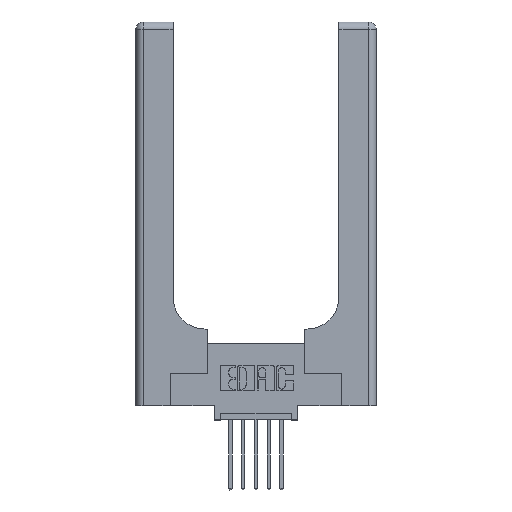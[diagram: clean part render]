
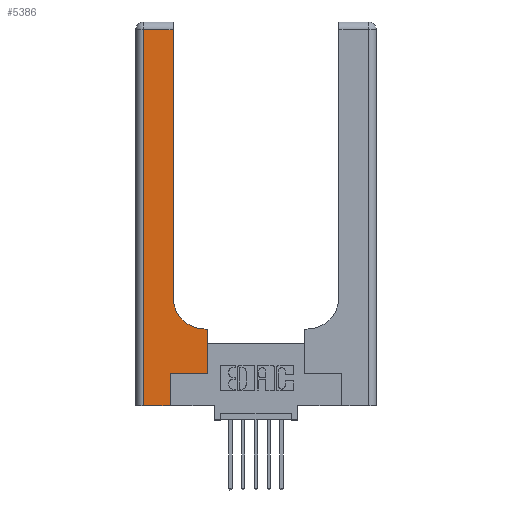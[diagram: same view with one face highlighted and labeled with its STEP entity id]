
A CAD part, top view. The second image highlights one B-rep face of the part: STEP entity #5386.
In plain terms, the highlighted planar face has unit normal (0, 0, 1).
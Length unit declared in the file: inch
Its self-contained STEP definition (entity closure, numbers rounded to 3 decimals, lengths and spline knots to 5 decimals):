
#36 = DIRECTION ( 'NONE',  ( 0., 1., 0. ) ) ;
#303 = CARTESIAN_POINT ( 'NONE',  ( 0.06, 3., 0.37 ) ) ;
#1174 = EDGE_CURVE ( 'NONE', #7339, #3521, #2783, .T. ) ;
#1209 = CARTESIAN_POINT ( 'NONE',  ( 0.06, 0., 0.37 ) ) ;
#1458 = CARTESIAN_POINT ( 'NONE',  ( 0.5585, 0.6, 0.37 ) ) ;
#1649 = LINE ( 'NONE', #8675, #6538 ) ;
#1860 = DIRECTION ( 'NONE',  ( 1., 0., 0. ) ) ;
#1893 = VECTOR ( 'NONE', #12234, 39.37008 ) ;
#2196 = VERTEX_POINT ( 'NONE', #2600 ) ;
#2221 = EDGE_CURVE ( 'NONE', #11413, #2196, #4609, .T. ) ;
#2308 = EDGE_CURVE ( 'NONE', #9584, #7339, #8987, .T. ) ;
#2595 = ORIENTED_EDGE ( 'NONE', *, *, #2221, .T. ) ;
#2600 = CARTESIAN_POINT ( 'NONE',  ( 0.2915, 2.94, 0.37 ) ) ;
#2644 = EDGE_CURVE ( 'NONE', #13141, #11413, #7642, .T. ) ;
#2783 = LINE ( 'NONE', #12352, #10411 ) ;
#2870 = EDGE_CURVE ( 'NONE', #6357, #9584, #1649, .T. ) ;
#3113 = VECTOR ( 'NONE', #10806, 39.37008 ) ;
#3154 = CARTESIAN_POINT ( 'NONE',  ( 0.5585, 0.25, 0.37 ) ) ;
#3508 = EDGE_CURVE ( 'NONE', #14069, #12065, #7256, .T. ) ;
#3521 = VERTEX_POINT ( 'NONE', #1458 ) ;
#4535 = EDGE_CURVE ( 'NONE', #2196, #14069, #11646, .T. ) ;
#4609 = LINE ( 'NONE', #5843, #11893 ) ;
#4682 = DIRECTION ( 'NONE',  ( 0., 1., 0. ) ) ;
#4736 = CARTESIAN_POINT ( 'NONE',  ( 0.269, 0., 0.37 ) ) ;
#4805 = AXIS2_PLACEMENT_3D ( 'NONE', #6147, #7114, #1860 ) ;
#4985 = ORIENTED_EDGE ( 'NONE', *, *, #2644, .T. ) ;
#5265 = CARTESIAN_POINT ( 'NONE',  ( 0.2915, 0.6, 0.37 ) ) ;
#5320 = DIRECTION ( 'NONE',  ( 0., 0., -1. ) ) ;
#5386 = ADVANCED_FACE ( 'NONE', ( #8868 ), #7463, .F. ) ;
#5843 = CARTESIAN_POINT ( 'NONE',  ( 0.2915, 3., 0.37 ) ) ;
#5983 = ORIENTED_EDGE ( 'NONE', *, *, #14091, .T. ) ;
#6147 = CARTESIAN_POINT ( 'NONE',  ( 0.5415, 0.85, 0.37 ) ) ;
#6179 = ORIENTED_EDGE ( 'NONE', *, *, #2308, .T. ) ;
#6357 = VERTEX_POINT ( 'NONE', #4736 ) ;
#6538 = VECTOR ( 'NONE', #36, 39.37008 ) ;
#6541 = VECTOR ( 'NONE', #7870, 39.37008 ) ;
#6996 = CARTESIAN_POINT ( 'NONE',  ( 0., 0., 0.37 ) ) ;
#7114 = DIRECTION ( 'NONE',  ( 0., 0., -1. ) ) ;
#7230 = ORIENTED_EDGE ( 'NONE', *, *, #12200, .T. ) ;
#7256 = LINE ( 'NONE', #303, #6541 ) ;
#7306 = CARTESIAN_POINT ( 'NONE',  ( 0.06, 2.94, 0.37 ) ) ;
#7339 = VERTEX_POINT ( 'NONE', #3154 ) ;
#7463 = PLANE ( 'NONE',  #9279 ) ;
#7467 = EDGE_LOOP ( 'NONE', ( #2595, #8911, #13981, #7230, #11034, #6179, #11875, #5983, #4985 ) ) ;
#7642 = CIRCLE ( 'NONE', #4805, 0.25 ) ;
#7689 = CARTESIAN_POINT ( 'NONE',  ( 0., 2.94, 0.37 ) ) ;
#7870 = DIRECTION ( 'NONE',  ( 0., -1., 0. ) ) ;
#8197 = LINE ( 'NONE', #5265, #3113 ) ;
#8675 = CARTESIAN_POINT ( 'NONE',  ( 0.269, 0., 0.37 ) ) ;
#8716 = CARTESIAN_POINT ( 'NONE',  ( 0.2915, 0.85, 0.37 ) ) ;
#8868 = FACE_OUTER_BOUND ( 'NONE', #7467, .T. ) ;
#8911 = ORIENTED_EDGE ( 'NONE', *, *, #4535, .T. ) ;
#8987 = LINE ( 'NONE', #11306, #1893 ) ;
#9279 = AXIS2_PLACEMENT_3D ( 'NONE', #10775, #5320, #11216 ) ;
#9584 = VERTEX_POINT ( 'NONE', #13653 ) ;
#10411 = VECTOR ( 'NONE', #10550, 39.37008 ) ;
#10550 = DIRECTION ( 'NONE',  ( 0., 1., 0. ) ) ;
#10775 = CARTESIAN_POINT ( 'NONE',  ( 0., 3., 0.37 ) ) ;
#10806 = DIRECTION ( 'NONE',  ( -1., 0., 0. ) ) ;
#11034 = ORIENTED_EDGE ( 'NONE', *, *, #2870, .T. ) ;
#11216 = DIRECTION ( 'NONE',  ( -1., 0., 0. ) ) ;
#11306 = CARTESIAN_POINT ( 'NONE',  ( 0.269, 0.25, 0.37 ) ) ;
#11413 = VERTEX_POINT ( 'NONE', #8716 ) ;
#11646 = LINE ( 'NONE', #7689, #11794 ) ;
#11650 = VECTOR ( 'NONE', #13497, 39.37008 ) ;
#11794 = VECTOR ( 'NONE', #13369, 39.37008 ) ;
#11875 = ORIENTED_EDGE ( 'NONE', *, *, #1174, .T. ) ;
#11893 = VECTOR ( 'NONE', #4682, 39.37008 ) ;
#12065 = VERTEX_POINT ( 'NONE', #1209 ) ;
#12088 = CARTESIAN_POINT ( 'NONE',  ( 0.5415, 0.6, 0.37 ) ) ;
#12200 = EDGE_CURVE ( 'NONE', #12065, #6357, #12965, .T. ) ;
#12234 = DIRECTION ( 'NONE',  ( 1., 0., 0. ) ) ;
#12352 = CARTESIAN_POINT ( 'NONE',  ( 0.5585, 0.25, 0.37 ) ) ;
#12965 = LINE ( 'NONE', #6996, #11650 ) ;
#13141 = VERTEX_POINT ( 'NONE', #12088 ) ;
#13369 = DIRECTION ( 'NONE',  ( -1., 0., 0. ) ) ;
#13497 = DIRECTION ( 'NONE',  ( 1., 0., 0. ) ) ;
#13653 = CARTESIAN_POINT ( 'NONE',  ( 0.269, 0.25, 0.37 ) ) ;
#13981 = ORIENTED_EDGE ( 'NONE', *, *, #3508, .T. ) ;
#14069 = VERTEX_POINT ( 'NONE', #7306 ) ;
#14091 = EDGE_CURVE ( 'NONE', #3521, #13141, #8197, .T. ) ;
